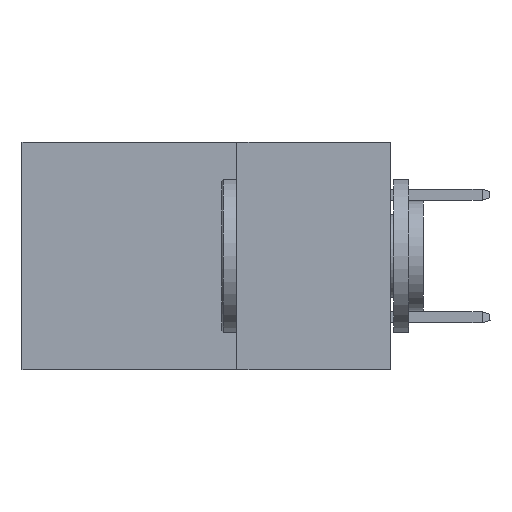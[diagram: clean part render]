
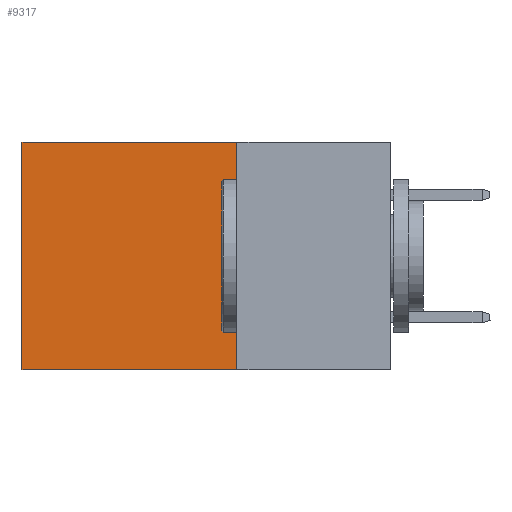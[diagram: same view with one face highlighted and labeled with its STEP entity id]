
A CAD part, left-side view. The second image highlights one B-rep face of the part: STEP entity #9317.
In plain terms, the highlighted planar face has unit normal (-1, 0, 0).
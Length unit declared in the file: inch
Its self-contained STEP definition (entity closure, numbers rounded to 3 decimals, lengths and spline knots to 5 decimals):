
#3 = EDGE_CURVE ( 'NONE', #24006, #1190, #5594, .T. ) ;
#142 = ORIENTED_EDGE ( 'NONE', *, *, #3, .T. ) ;
#1190 = VERTEX_POINT ( 'NONE', #24394 ) ;
#1812 = VECTOR ( 'NONE', #13551, 39.37008 ) ;
#2919 = CARTESIAN_POINT ( 'NONE',  ( 0.2875, 0.6, 0. ) ) ;
#3068 = EDGE_CURVE ( 'NONE', #1190, #7917, #7077, .T. ) ;
#3735 = LINE ( 'NONE', #14413, #9671 ) ;
#4614 = VECTOR ( 'NONE', #25836, 39.37008 ) ;
#5022 = ORIENTED_EDGE ( 'NONE', *, *, #20722, .F. ) ;
#5594 = LINE ( 'NONE', #5624, #8886 ) ;
#5624 = CARTESIAN_POINT ( 'NONE',  ( 0.2875, 0.25, 0. ) ) ;
#6935 = CARTESIAN_POINT ( 'NONE',  ( 0.2875, 0.25, -0.37 ) ) ;
#6992 = EDGE_LOOP ( 'NONE', ( #17985, #5022, #23760, #142 ) ) ;
#7077 = LINE ( 'NONE', #2919, #1812 ) ;
#7917 = VERTEX_POINT ( 'NONE', #20964 ) ;
#8886 = VECTOR ( 'NONE', #25612, 39.37008 ) ;
#9050 = EDGE_CURVE ( 'NONE', #24006, #20838, #3735, .T. ) ;
#9317 = ADVANCED_FACE ( 'NONE', ( #11914 ), #22734, .F. ) ;
#9671 = VECTOR ( 'NONE', #10201, 39.37008 ) ;
#9831 = CARTESIAN_POINT ( 'NONE',  ( 0.2875, 0.25, 0. ) ) ;
#10201 = DIRECTION ( 'NONE',  ( 0., 0., -1. ) ) ;
#11914 = FACE_OUTER_BOUND ( 'NONE', #6992, .T. ) ;
#11980 = DIRECTION ( 'NONE',  ( 1., 0., 0. ) ) ;
#13551 = DIRECTION ( 'NONE',  ( 0., 0., -1. ) ) ;
#14413 = CARTESIAN_POINT ( 'NONE',  ( 0.2875, 0.25, 0. ) ) ;
#15006 = CARTESIAN_POINT ( 'NONE',  ( 0.2875, 0.25, 0. ) ) ;
#17985 = ORIENTED_EDGE ( 'NONE', *, *, #3068, .T. ) ;
#19677 = CARTESIAN_POINT ( 'NONE',  ( 0.2875, 0.25, -0.37 ) ) ;
#20722 = EDGE_CURVE ( 'NONE', #20838, #7917, #24686, .T. ) ;
#20838 = VERTEX_POINT ( 'NONE', #19677 ) ;
#20964 = CARTESIAN_POINT ( 'NONE',  ( 0.2875, 0.6, -0.37 ) ) ;
#22373 = DIRECTION ( 'NONE',  ( 0., 0., -1. ) ) ;
#22734 = PLANE ( 'NONE',  #25654 ) ;
#23760 = ORIENTED_EDGE ( 'NONE', *, *, #9050, .F. ) ;
#24006 = VERTEX_POINT ( 'NONE', #15006 ) ;
#24394 = CARTESIAN_POINT ( 'NONE',  ( 0.2875, 0.6, 0. ) ) ;
#24686 = LINE ( 'NONE', #6935, #4614 ) ;
#25612 = DIRECTION ( 'NONE',  ( 0., 1., 0. ) ) ;
#25654 = AXIS2_PLACEMENT_3D ( 'NONE', #9831, #11980, #22373 ) ;
#25836 = DIRECTION ( 'NONE',  ( 0., 1., 0. ) ) ;
